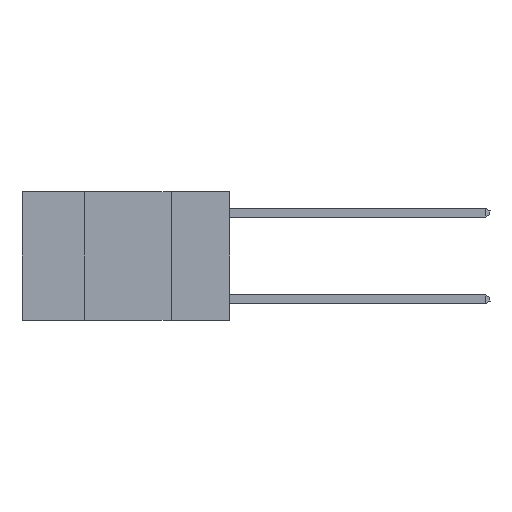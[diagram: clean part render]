
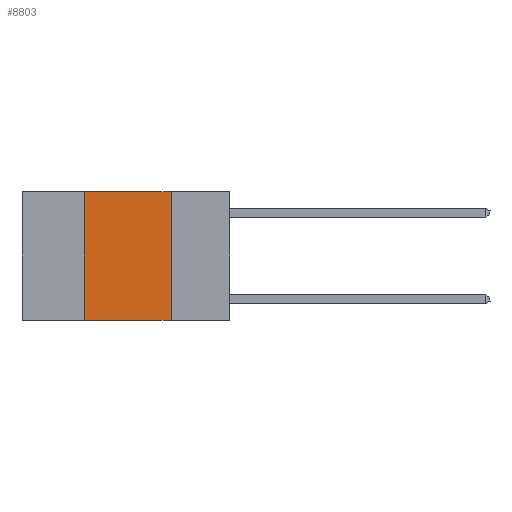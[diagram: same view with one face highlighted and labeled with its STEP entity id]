
A CAD part, left-side view. The second image highlights one B-rep face of the part: STEP entity #8803.
In plain terms, the highlighted planar face has unit normal (-1, 0, 0).
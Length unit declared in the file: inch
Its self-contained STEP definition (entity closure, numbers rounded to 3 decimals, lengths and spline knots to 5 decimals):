
#122 = VECTOR ( 'NONE', #622, 39.37008 ) ;
#349 = EDGE_CURVE ( 'NONE', #6174, #12720, #10026, .T. ) ;
#598 = CARTESIAN_POINT ( 'NONE',  ( 0., 0.6, 0. ) ) ;
#622 = DIRECTION ( 'NONE',  ( 0., -1., 0. ) ) ;
#1122 = EDGE_CURVE ( 'NONE', #8226, #6796, #4427, .T. ) ;
#1207 = EDGE_CURVE ( 'NONE', #12720, #8226, #10152, .T. ) ;
#2699 = VECTOR ( 'NONE', #3581, 39.37008 ) ;
#2874 = DIRECTION ( 'NONE',  ( 1., 0., 0. ) ) ;
#3448 = CARTESIAN_POINT ( 'NONE',  ( 0., 0.17, 0. ) ) ;
#3581 = DIRECTION ( 'NONE',  ( 0., -1., 0. ) ) ;
#3833 = CARTESIAN_POINT ( 'NONE',  ( 0., 0.42, 0. ) ) ;
#4427 = LINE ( 'NONE', #3448, #9384 ) ;
#4724 = ORIENTED_EDGE ( 'NONE', *, *, #10409, .T. ) ;
#5425 = CARTESIAN_POINT ( 'NONE',  ( 0., 0.42, -0.37 ) ) ;
#5997 = CARTESIAN_POINT ( 'NONE',  ( 0., 0.17, 0. ) ) ;
#6174 = VERTEX_POINT ( 'NONE', #5425 ) ;
#6452 = CARTESIAN_POINT ( 'NONE',  ( 0., 0.42, 0. ) ) ;
#6796 = VERTEX_POINT ( 'NONE', #7626 ) ;
#7122 = DIRECTION ( 'NONE',  ( 0., 0., -1. ) ) ;
#7626 = CARTESIAN_POINT ( 'NONE',  ( 0., 0.17, -0.37 ) ) ;
#8169 = PLANE ( 'NONE',  #11855 ) ;
#8226 = VERTEX_POINT ( 'NONE', #5997 ) ;
#8781 = ORIENTED_EDGE ( 'NONE', *, *, #349, .F. ) ;
#8803 = ADVANCED_FACE ( 'NONE', ( #11148 ), #8169, .F. ) ;
#9384 = VECTOR ( 'NONE', #11956, 39.37008 ) ;
#9596 = VECTOR ( 'NONE', #12341, 39.37008 ) ;
#10026 = LINE ( 'NONE', #3833, #9596 ) ;
#10152 = LINE ( 'NONE', #598, #2699 ) ;
#10269 = ORIENTED_EDGE ( 'NONE', *, *, #1122, .F. ) ;
#10409 = EDGE_CURVE ( 'NONE', #6174, #6796, #12122, .T. ) ;
#10463 = EDGE_LOOP ( 'NONE', ( #10269, #12731, #8781, #4724 ) ) ;
#11084 = CARTESIAN_POINT ( 'NONE',  ( 0., 0.6, 0. ) ) ;
#11148 = FACE_OUTER_BOUND ( 'NONE', #10463, .T. ) ;
#11855 = AXIS2_PLACEMENT_3D ( 'NONE', #11084, #2874, #7122 ) ;
#11956 = DIRECTION ( 'NONE',  ( 0., 0., -1. ) ) ;
#12122 = LINE ( 'NONE', #13216, #122 ) ;
#12341 = DIRECTION ( 'NONE',  ( 0., 0., 1. ) ) ;
#12720 = VERTEX_POINT ( 'NONE', #6452 ) ;
#12731 = ORIENTED_EDGE ( 'NONE', *, *, #1207, .F. ) ;
#13216 = CARTESIAN_POINT ( 'NONE',  ( 0., 0.6, -0.37 ) ) ;
